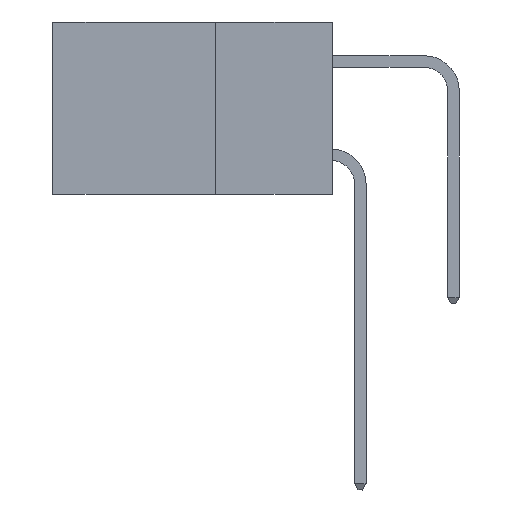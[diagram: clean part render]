
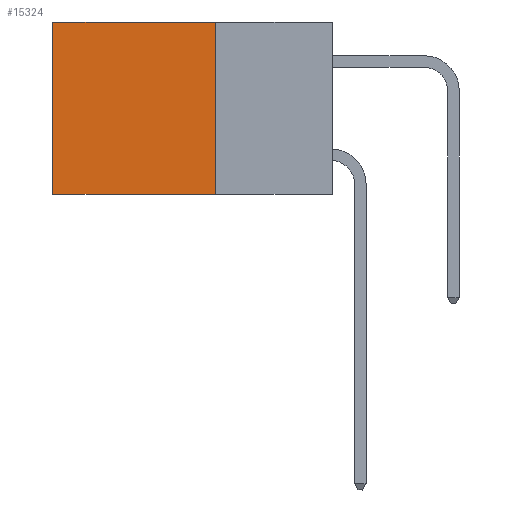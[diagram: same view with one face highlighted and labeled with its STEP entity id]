
A CAD part, left-side view. The second image highlights one B-rep face of the part: STEP entity #15324.
In plain terms, the highlighted planar face has unit normal (-1, 0, 0).
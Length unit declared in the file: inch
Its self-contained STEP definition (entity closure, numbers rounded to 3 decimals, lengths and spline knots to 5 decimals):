
#16 = VECTOR ( 'NONE', #4906, 39.37008 ) ;
#250 = DIRECTION ( 'NONE',  ( 0., 0., -1. ) ) ;
#461 = VECTOR ( 'NONE', #5488, 39.37008 ) ;
#463 = ORIENTED_EDGE ( 'NONE', *, *, #8493, .F. ) ;
#679 = VERTEX_POINT ( 'NONE', #1013 ) ;
#842 = EDGE_CURVE ( 'NONE', #5168, #14092, #6955, .T. ) ;
#1013 = CARTESIAN_POINT ( 'NONE',  ( 0.298, 0.6, 0. ) ) ;
#1201 = FACE_OUTER_BOUND ( 'NONE', #6829, .T. ) ;
#1503 = DIRECTION ( 'NONE',  ( 0., 1., 0. ) ) ;
#1627 = LINE ( 'NONE', #7677, #13611 ) ;
#2078 = CARTESIAN_POINT ( 'NONE',  ( 0.298, 0.6, -0.37 ) ) ;
#2456 = EDGE_CURVE ( 'NONE', #679, #11534, #13235, .T. ) ;
#2583 = EDGE_CURVE ( 'NONE', #5168, #679, #14146, .T. ) ;
#4359 = AXIS2_PLACEMENT_3D ( 'NONE', #13462, #7547, #250 ) ;
#4906 = DIRECTION ( 'NONE',  ( 0., 0., -1. ) ) ;
#5135 = PLANE ( 'NONE',  #4359 ) ;
#5168 = VERTEX_POINT ( 'NONE', #11606 ) ;
#5488 = DIRECTION ( 'NONE',  ( 0., 0., -1. ) ) ;
#5757 = ORIENTED_EDGE ( 'NONE', *, *, #2583, .T. ) ;
#6742 = ORIENTED_EDGE ( 'NONE', *, *, #842, .F. ) ;
#6829 = EDGE_LOOP ( 'NONE', ( #12088, #463, #6742, #5757 ) ) ;
#6955 = LINE ( 'NONE', #15317, #461 ) ;
#7547 = DIRECTION ( 'NONE',  ( 1., 0., 0. ) ) ;
#7677 = CARTESIAN_POINT ( 'NONE',  ( 0.298, 0.25, -0.37 ) ) ;
#8493 = EDGE_CURVE ( 'NONE', #14092, #11534, #1627, .T. ) ;
#8741 = CARTESIAN_POINT ( 'NONE',  ( 0.298, 0.25, 0. ) ) ;
#8889 = DIRECTION ( 'NONE',  ( 0., 1., 0. ) ) ;
#10891 = CARTESIAN_POINT ( 'NONE',  ( 0.298, 0.6, 0. ) ) ;
#11534 = VERTEX_POINT ( 'NONE', #2078 ) ;
#11606 = CARTESIAN_POINT ( 'NONE',  ( 0.298, 0.25, 0. ) ) ;
#12088 = ORIENTED_EDGE ( 'NONE', *, *, #2456, .T. ) ;
#12159 = VECTOR ( 'NONE', #1503, 39.37008 ) ;
#13235 = LINE ( 'NONE', #10891, #16 ) ;
#13462 = CARTESIAN_POINT ( 'NONE',  ( 0.298, 0.25, 0. ) ) ;
#13611 = VECTOR ( 'NONE', #8889, 39.37008 ) ;
#14092 = VERTEX_POINT ( 'NONE', #15402 ) ;
#14146 = LINE ( 'NONE', #8741, #12159 ) ;
#15317 = CARTESIAN_POINT ( 'NONE',  ( 0.298, 0.25, 0. ) ) ;
#15324 = ADVANCED_FACE ( 'NONE', ( #1201 ), #5135, .F. ) ;
#15402 = CARTESIAN_POINT ( 'NONE',  ( 0.298, 0.25, -0.37 ) ) ;
